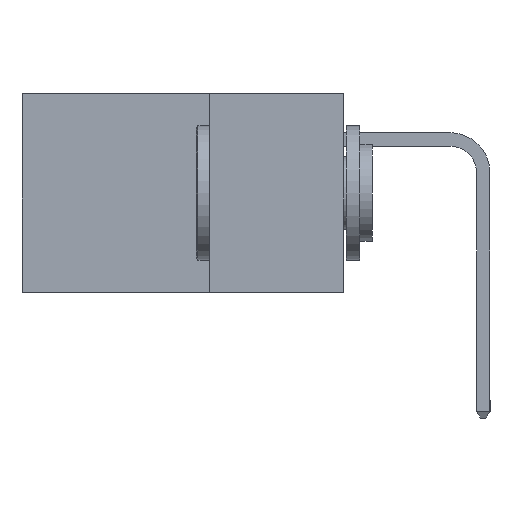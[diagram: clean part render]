
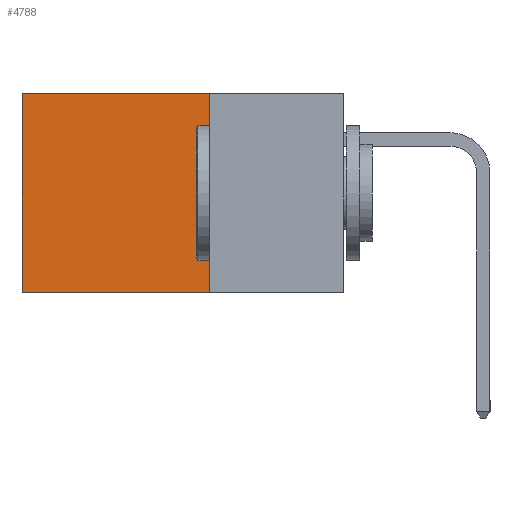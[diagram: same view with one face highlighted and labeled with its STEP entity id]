
A CAD part, left-side view. The second image highlights one B-rep face of the part: STEP entity #4788.
In plain terms, the highlighted planar face has unit normal (-1, 0, 0).
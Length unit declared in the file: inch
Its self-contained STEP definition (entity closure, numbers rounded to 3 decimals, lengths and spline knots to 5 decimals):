
#28 = ORIENTED_EDGE ( 'NONE', *, *, #9882, .T. ) ;
#1888 = VECTOR ( 'NONE', #4805, 39.37008 ) ;
#2104 = EDGE_CURVE ( 'NONE', #9201, #3207, #12801, .T. ) ;
#2804 = DIRECTION ( 'NONE',  ( 0., 0., -1. ) ) ;
#2969 = LINE ( 'NONE', #3592, #9128 ) ;
#3149 = EDGE_CURVE ( 'NONE', #11571, #3207, #13710, .T. ) ;
#3207 = VERTEX_POINT ( 'NONE', #5677 ) ;
#3549 = CARTESIAN_POINT ( 'NONE',  ( 0.2615, 0.25, -0.37 ) ) ;
#3592 = CARTESIAN_POINT ( 'NONE',  ( 0.2615, 0.25, 0. ) ) ;
#3984 = VECTOR ( 'NONE', #6021, 39.37008 ) ;
#4788 = ADVANCED_FACE ( 'NONE', ( #9715 ), #6680, .F. ) ;
#4805 = DIRECTION ( 'NONE',  ( 0., 0., -1. ) ) ;
#5318 = CARTESIAN_POINT ( 'NONE',  ( 0.2615, 0.25, -0.37 ) ) ;
#5677 = CARTESIAN_POINT ( 'NONE',  ( 0.2615, 0.6, -0.37 ) ) ;
#6017 = VERTEX_POINT ( 'NONE', #8252 ) ;
#6021 = DIRECTION ( 'NONE',  ( 0., 1., 0. ) ) ;
#6048 = DIRECTION ( 'NONE',  ( 0., 1., 0. ) ) ;
#6056 = CARTESIAN_POINT ( 'NONE',  ( 0.2615, 0.25, -0.37 ) ) ;
#6487 = AXIS2_PLACEMENT_3D ( 'NONE', #7026, #6904, #2804 ) ;
#6680 = PLANE ( 'NONE',  #6487 ) ;
#6904 = DIRECTION ( 'NONE',  ( 1., 0., 0. ) ) ;
#7026 = CARTESIAN_POINT ( 'NONE',  ( 0.2615, 0.25, -0.37 ) ) ;
#7826 = ORIENTED_EDGE ( 'NONE', *, *, #13274, .F. ) ;
#8252 = CARTESIAN_POINT ( 'NONE',  ( 0.2615, 0.25, 0. ) ) ;
#9128 = VECTOR ( 'NONE', #6048, 39.37008 ) ;
#9199 = VECTOR ( 'NONE', #14746, 39.37008 ) ;
#9201 = VERTEX_POINT ( 'NONE', #15740 ) ;
#9715 = FACE_OUTER_BOUND ( 'NONE', #10152, .T. ) ;
#9882 = EDGE_CURVE ( 'NONE', #6017, #9201, #2969, .T. ) ;
#10004 = ORIENTED_EDGE ( 'NONE', *, *, #2104, .T. ) ;
#10152 = EDGE_LOOP ( 'NONE', ( #10004, #15561, #7826, #28 ) ) ;
#11571 = VERTEX_POINT ( 'NONE', #5318 ) ;
#11671 = LINE ( 'NONE', #3549, #1888 ) ;
#12801 = LINE ( 'NONE', #14794, #9199 ) ;
#13274 = EDGE_CURVE ( 'NONE', #6017, #11571, #11671, .T. ) ;
#13710 = LINE ( 'NONE', #6056, #3984 ) ;
#14746 = DIRECTION ( 'NONE',  ( 0., 0., -1. ) ) ;
#14794 = CARTESIAN_POINT ( 'NONE',  ( 0.2615, 0.6, -0.37 ) ) ;
#15561 = ORIENTED_EDGE ( 'NONE', *, *, #3149, .F. ) ;
#15740 = CARTESIAN_POINT ( 'NONE',  ( 0.2615, 0.6, 0. ) ) ;
